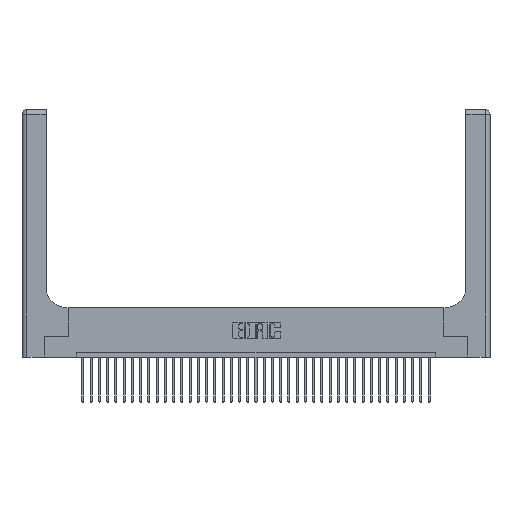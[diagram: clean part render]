
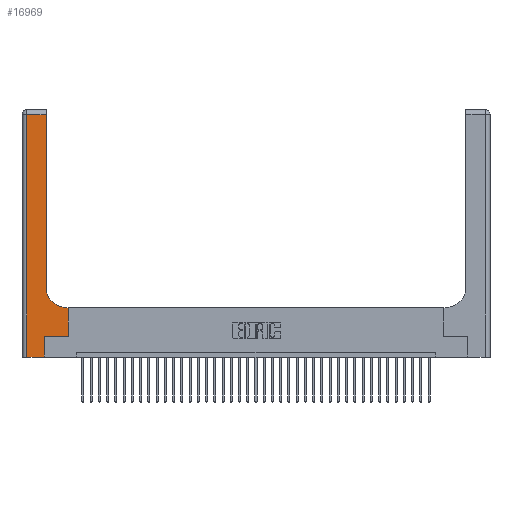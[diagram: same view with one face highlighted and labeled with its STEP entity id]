
A CAD part, top view. The second image highlights one B-rep face of the part: STEP entity #16969.
In plain terms, the highlighted planar face has unit normal (0, 0, 1).
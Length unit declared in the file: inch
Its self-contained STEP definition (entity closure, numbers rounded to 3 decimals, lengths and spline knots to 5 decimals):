
#833 = CARTESIAN_POINT ( 'NONE',  ( 0., 3., 0.37 ) ) ;
#1507 = VERTEX_POINT ( 'NONE', #3386 ) ;
#2364 = EDGE_LOOP ( 'NONE', ( #29781, #9082, #2978, #35032, #21865, #22279, #36097, #15593, #36172 ) ) ;
#2378 = DIRECTION ( 'NONE',  ( 1., 0., 0. ) ) ;
#2978 = ORIENTED_EDGE ( 'NONE', *, *, #24922, .T. ) ;
#3386 = CARTESIAN_POINT ( 'NONE',  ( 0.269, 0., 0.37 ) ) ;
#4346 = DIRECTION ( 'NONE',  ( 0., 0., -1. ) ) ;
#4356 = VECTOR ( 'NONE', #34758, 39.37008 ) ;
#4543 = LINE ( 'NONE', #22169, #18098 ) ;
#4879 = EDGE_CURVE ( 'NONE', #5309, #7152, #10061, .T. ) ;
#5198 = VERTEX_POINT ( 'NONE', #30145 ) ;
#5309 = VERTEX_POINT ( 'NONE', #24182 ) ;
#5783 = EDGE_CURVE ( 'NONE', #23158, #16120, #14528, .T. ) ;
#7152 = VERTEX_POINT ( 'NONE', #12628 ) ;
#7685 = DIRECTION ( 'NONE',  ( 0., 1., 0. ) ) ;
#9082 = ORIENTED_EDGE ( 'NONE', *, *, #4879, .T. ) ;
#9252 = VECTOR ( 'NONE', #7685, 39.37008 ) ;
#9617 = CARTESIAN_POINT ( 'NONE',  ( 0.269, 0.25, 0.37 ) ) ;
#10061 = LINE ( 'NONE', #19434, #29999 ) ;
#10167 = DIRECTION ( 'NONE',  ( -1., 0., 0. ) ) ;
#10686 = DIRECTION ( 'NONE',  ( 0., 1., 0. ) ) ;
#11988 = LINE ( 'NONE', #12512, #4356 ) ;
#12129 = VECTOR ( 'NONE', #10167, 39.37008 ) ;
#12289 = DIRECTION ( 'NONE',  ( 0., 0., -1. ) ) ;
#12317 = LINE ( 'NONE', #13948, #19155 ) ;
#12512 = CARTESIAN_POINT ( 'NONE',  ( 0.06, 3., 0.37 ) ) ;
#12628 = CARTESIAN_POINT ( 'NONE',  ( 0.06, 2.94, 0.37 ) ) ;
#13171 = EDGE_CURVE ( 'NONE', #24544, #1507, #28412, .T. ) ;
#13948 = CARTESIAN_POINT ( 'NONE',  ( 0.269, 0.25, 0.37 ) ) ;
#14528 = CIRCLE ( 'NONE', #34951, 0.25 ) ;
#15564 = AXIS2_PLACEMENT_3D ( 'NONE', #833, #12289, #32559 ) ;
#15593 = ORIENTED_EDGE ( 'NONE', *, *, #22670, .T. ) ;
#16091 = EDGE_CURVE ( 'NONE', #16120, #5309, #21790, .T. ) ;
#16120 = VERTEX_POINT ( 'NONE', #19556 ) ;
#16411 = EDGE_CURVE ( 'NONE', #5198, #21747, #4543, .T. ) ;
#16664 = CARTESIAN_POINT ( 'NONE',  ( 0.2915, 3., 0.37 ) ) ;
#16969 = ADVANCED_FACE ( 'NONE', ( #18525 ), #18005, .F. ) ;
#17019 = DIRECTION ( 'NONE',  ( -1., 0., 0. ) ) ;
#18005 = PLANE ( 'NONE',  #15564 ) ;
#18040 = CARTESIAN_POINT ( 'NONE',  ( 0.269, 0., 0.37 ) ) ;
#18098 = VECTOR ( 'NONE', #21812, 39.37008 ) ;
#18525 = FACE_OUTER_BOUND ( 'NONE', #2364, .T. ) ;
#19155 = VECTOR ( 'NONE', #19537, 39.37008 ) ;
#19434 = CARTESIAN_POINT ( 'NONE',  ( 0., 2.94, 0.37 ) ) ;
#19537 = DIRECTION ( 'NONE',  ( 1., 0., 0. ) ) ;
#19556 = CARTESIAN_POINT ( 'NONE',  ( 0.2915, 0.85, 0.37 ) ) ;
#19690 = CARTESIAN_POINT ( 'NONE',  ( 0., 0., 0.37 ) ) ;
#21747 = VERTEX_POINT ( 'NONE', #36649 ) ;
#21790 = LINE ( 'NONE', #16664, #23999 ) ;
#21812 = DIRECTION ( 'NONE',  ( 0., 1., 0. ) ) ;
#21865 = ORIENTED_EDGE ( 'NONE', *, *, #25090, .T. ) ;
#21946 = CARTESIAN_POINT ( 'NONE',  ( 0.2915, 0.6, 0.37 ) ) ;
#22169 = CARTESIAN_POINT ( 'NONE',  ( 0.5585, 0.25, 0.37 ) ) ;
#22279 = ORIENTED_EDGE ( 'NONE', *, *, #25998, .T. ) ;
#22670 = EDGE_CURVE ( 'NONE', #21747, #23158, #26145, .T. ) ;
#23158 = VERTEX_POINT ( 'NONE', #26792 ) ;
#23704 = LINE ( 'NONE', #18040, #9252 ) ;
#23819 = VECTOR ( 'NONE', #2378, 39.37008 ) ;
#23999 = VECTOR ( 'NONE', #10686, 39.37008 ) ;
#24182 = CARTESIAN_POINT ( 'NONE',  ( 0.2915, 2.94, 0.37 ) ) ;
#24544 = VERTEX_POINT ( 'NONE', #32599 ) ;
#24922 = EDGE_CURVE ( 'NONE', #7152, #24544, #11988, .T. ) ;
#25090 = EDGE_CURVE ( 'NONE', #1507, #33406, #23704, .T. ) ;
#25998 = EDGE_CURVE ( 'NONE', #33406, #5198, #12317, .T. ) ;
#26145 = LINE ( 'NONE', #21946, #12129 ) ;
#26792 = CARTESIAN_POINT ( 'NONE',  ( 0.5415, 0.6, 0.37 ) ) ;
#28412 = LINE ( 'NONE', #19690, #23819 ) ;
#29781 = ORIENTED_EDGE ( 'NONE', *, *, #16091, .T. ) ;
#29999 = VECTOR ( 'NONE', #17019, 39.37008 ) ;
#30145 = CARTESIAN_POINT ( 'NONE',  ( 0.5585, 0.25, 0.37 ) ) ;
#32559 = DIRECTION ( 'NONE',  ( -1., 0., 0. ) ) ;
#32599 = CARTESIAN_POINT ( 'NONE',  ( 0.06, 0., 0.37 ) ) ;
#33406 = VERTEX_POINT ( 'NONE', #9617 ) ;
#34758 = DIRECTION ( 'NONE',  ( 0., -1., 0. ) ) ;
#34951 = AXIS2_PLACEMENT_3D ( 'NONE', #36699, #4346, #35479 ) ;
#35032 = ORIENTED_EDGE ( 'NONE', *, *, #13171, .T. ) ;
#35479 = DIRECTION ( 'NONE',  ( 1., 0., 0. ) ) ;
#36097 = ORIENTED_EDGE ( 'NONE', *, *, #16411, .T. ) ;
#36172 = ORIENTED_EDGE ( 'NONE', *, *, #5783, .T. ) ;
#36649 = CARTESIAN_POINT ( 'NONE',  ( 0.5585, 0.6, 0.37 ) ) ;
#36699 = CARTESIAN_POINT ( 'NONE',  ( 0.5415, 0.85, 0.37 ) ) ;
